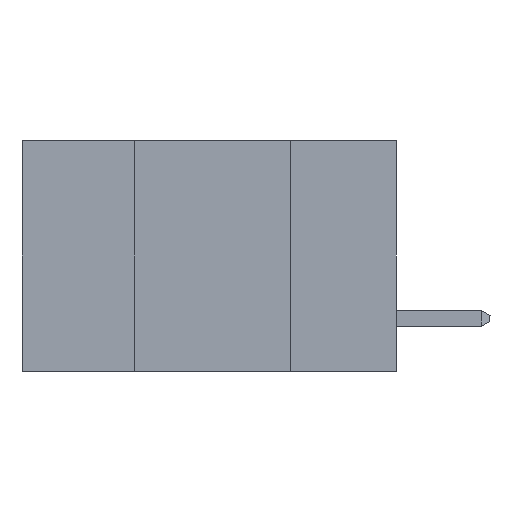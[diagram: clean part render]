
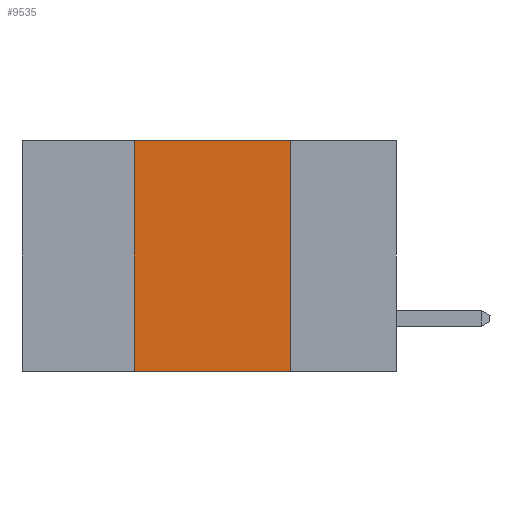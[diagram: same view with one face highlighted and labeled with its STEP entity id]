
A CAD part, left-side view. The second image highlights one B-rep face of the part: STEP entity #9535.
In plain terms, the highlighted planar face has unit normal (-1, 0, 0).
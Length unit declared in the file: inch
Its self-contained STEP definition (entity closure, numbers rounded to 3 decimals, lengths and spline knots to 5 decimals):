
#406 = ORIENTED_EDGE ( 'NONE', *, *, #2142, .F. ) ;
#423 = EDGE_CURVE ( 'NONE', #9492, #7094, #10340, .T. ) ;
#891 = DIRECTION ( 'NONE',  ( 0., -1., 0. ) ) ;
#944 = CARTESIAN_POINT ( 'NONE',  ( 0., 0.17, -0.37 ) ) ;
#1200 = ORIENTED_EDGE ( 'NONE', *, *, #7990, .F. ) ;
#1241 = EDGE_CURVE ( 'NONE', #4893, #7094, #1639, .T. ) ;
#1639 = LINE ( 'NONE', #6923, #3353 ) ;
#2142 = EDGE_CURVE ( 'NONE', #4893, #7541, #11112, .T. ) ;
#2803 = VECTOR ( 'NONE', #3444, 39.37008 ) ;
#2883 = DIRECTION ( 'NONE',  ( 0., 0., 1. ) ) ;
#3353 = VECTOR ( 'NONE', #891, 39.37008 ) ;
#3444 = DIRECTION ( 'NONE',  ( 0., -1., 0. ) ) ;
#3674 = CARTESIAN_POINT ( 'NONE',  ( 0., 0.6, 0. ) ) ;
#4816 = AXIS2_PLACEMENT_3D ( 'NONE', #3674, #9713, #5668 ) ;
#4893 = VERTEX_POINT ( 'NONE', #9626 ) ;
#5562 = CARTESIAN_POINT ( 'NONE',  ( 0., 0.17, -0.37 ) ) ;
#5563 = ORIENTED_EDGE ( 'NONE', *, *, #1241, .T. ) ;
#5668 = DIRECTION ( 'NONE',  ( 0., 0., -1. ) ) ;
#5850 = LINE ( 'NONE', #12830, #2803 ) ;
#5948 = EDGE_LOOP ( 'NONE', ( #8794, #1200, #406, #5563 ) ) ;
#6450 = VECTOR ( 'NONE', #2883, 39.37008 ) ;
#6923 = CARTESIAN_POINT ( 'NONE',  ( 0., 0.6, -0.37 ) ) ;
#7094 = VERTEX_POINT ( 'NONE', #5562 ) ;
#7541 = VERTEX_POINT ( 'NONE', #9024 ) ;
#7990 = EDGE_CURVE ( 'NONE', #7541, #9492, #5850, .T. ) ;
#8042 = CARTESIAN_POINT ( 'NONE',  ( 0., 0.42, -0.37 ) ) ;
#8616 = VECTOR ( 'NONE', #10543, 39.37008 ) ;
#8794 = ORIENTED_EDGE ( 'NONE', *, *, #423, .F. ) ;
#9024 = CARTESIAN_POINT ( 'NONE',  ( 0., 0.42, 0. ) ) ;
#9492 = VERTEX_POINT ( 'NONE', #12784 ) ;
#9535 = ADVANCED_FACE ( 'NONE', ( #10803 ), #10934, .F. ) ;
#9626 = CARTESIAN_POINT ( 'NONE',  ( 0., 0.42, -0.37 ) ) ;
#9713 = DIRECTION ( 'NONE',  ( 1., 0., 0. ) ) ;
#10340 = LINE ( 'NONE', #944, #8616 ) ;
#10543 = DIRECTION ( 'NONE',  ( 0., 0., -1. ) ) ;
#10803 = FACE_OUTER_BOUND ( 'NONE', #5948, .T. ) ;
#10934 = PLANE ( 'NONE',  #4816 ) ;
#11112 = LINE ( 'NONE', #8042, #6450 ) ;
#12784 = CARTESIAN_POINT ( 'NONE',  ( 0., 0.17, 0. ) ) ;
#12830 = CARTESIAN_POINT ( 'NONE',  ( 0., 0.6, 0. ) ) ;
